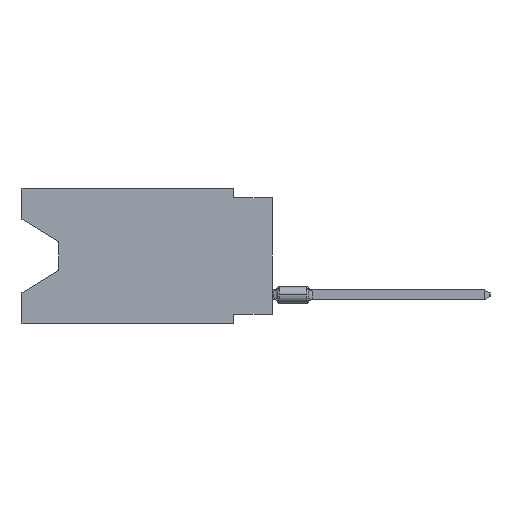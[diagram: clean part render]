
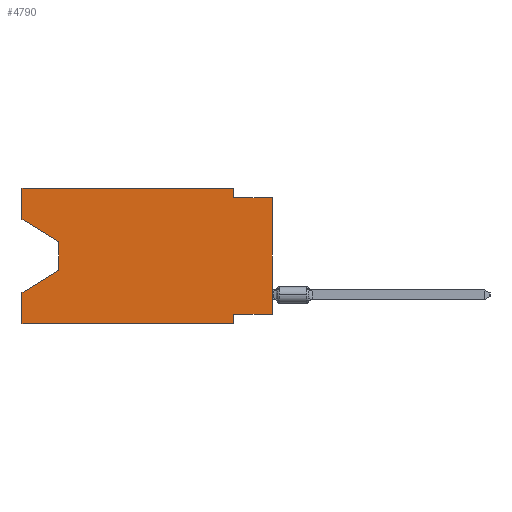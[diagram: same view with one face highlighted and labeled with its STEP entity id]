
A CAD part, left-side view. The second image highlights one B-rep face of the part: STEP entity #4790.
In plain terms, the highlighted planar face has unit normal (-1, 0, 0).
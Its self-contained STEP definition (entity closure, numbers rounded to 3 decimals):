
#1684 = DIRECTION ( 'NONE',  ( 0., -1., 0. ) ) ;
#2310 = VECTOR ( 'NONE', #32259, 1000. ) ;
#2344 = VERTEX_POINT ( 'NONE', #59910 ) ;
#2528 = CARTESIAN_POINT ( 'NONE',  ( 0., 16.383, 0. ) ) ;
#3266 = CARTESIAN_POINT ( 'NONE',  ( 0., 16.383, 0. ) ) ;
#3654 = CARTESIAN_POINT ( 'NONE',  ( 0., 16.383, 0. ) ) ;
#3919 = DIRECTION ( 'NONE',  ( 0., 0., 1. ) ) ;
#4790 = ADVANCED_FACE ( 'NONE', ( #25564 ), #44043, .F. ) ;
#5219 = ORIENTED_EDGE ( 'NONE', *, *, #53636, .F. ) ;
#5484 = VECTOR ( 'NONE', #18317, 1000. ) ;
#5953 = VERTEX_POINT ( 'NONE', #3266 ) ;
#6232 = LINE ( 'NONE', #38947, #46219 ) ;
#6606 = VERTEX_POINT ( 'NONE', #14410 ) ;
#6615 = CARTESIAN_POINT ( 'NONE',  ( 0., 16.383, 0. ) ) ;
#6878 = ORIENTED_EDGE ( 'NONE', *, *, #52395, .F. ) ;
#7997 = DIRECTION ( 'NONE',  ( 0., 1., 0. ) ) ;
#8465 = VERTEX_POINT ( 'NONE', #28831 ) ;
#8543 = CARTESIAN_POINT ( 'NONE',  ( 0., 2.54, -0.635 ) ) ;
#8695 = VECTOR ( 'NONE', #53645, 1000. ) ;
#8993 = CARTESIAN_POINT ( 'NONE',  ( 0., 16.383, 0. ) ) ;
#9482 = DIRECTION ( 'NONE',  ( 0., -0.855, -0.519 ) ) ;
#9536 = VECTOR ( 'NONE', #13551, 1000. ) ;
#10399 = ORIENTED_EDGE ( 'NONE', *, *, #22280, .T. ) ;
#10904 = ORIENTED_EDGE ( 'NONE', *, *, #12174, .F. ) ;
#11499 = VECTOR ( 'NONE', #42005, 1000. ) ;
#11613 = AXIS2_PLACEMENT_3D ( 'NONE', #2528, #21022, #39489 ) ;
#12174 = EDGE_CURVE ( 'NONE', #33151, #37188, #49015, .T. ) ;
#12844 = LINE ( 'NONE', #54327, #21352 ) ;
#13045 = LINE ( 'NONE', #3654, #8695 ) ;
#13262 = CARTESIAN_POINT ( 'NONE',  ( 0., 16.383, -2.038 ) ) ;
#13551 = DIRECTION ( 'NONE',  ( 0., 0.855, -0.519 ) ) ;
#14410 = CARTESIAN_POINT ( 'NONE',  ( 0., 0., -8.255 ) ) ;
#15656 = CARTESIAN_POINT ( 'NONE',  ( 0., 0., -0.635 ) ) ;
#16325 = DIRECTION ( 'NONE',  ( 0., 0., 1. ) ) ;
#16376 = ORIENTED_EDGE ( 'NONE', *, *, #46644, .F. ) ;
#18317 = DIRECTION ( 'NONE',  ( 0., 0., -1. ) ) ;
#18610 = CARTESIAN_POINT ( 'NONE',  ( 0., 2.54, 0. ) ) ;
#19318 = ORIENTED_EDGE ( 'NONE', *, *, #20815, .F. ) ;
#20003 = VERTEX_POINT ( 'NONE', #24184 ) ;
#20815 = EDGE_CURVE ( 'NONE', #23128, #49265, #54342, .T. ) ;
#21022 = DIRECTION ( 'NONE',  ( 1., 0., 0. ) ) ;
#21352 = VECTOR ( 'NONE', #7997, 1000. ) ;
#22280 = EDGE_CURVE ( 'NONE', #33151, #55894, #6232, .T. ) ;
#22934 = CARTESIAN_POINT ( 'NONE',  ( 0., 13.97, -5.385 ) ) ;
#23128 = VERTEX_POINT ( 'NONE', #39033 ) ;
#23305 = EDGE_CURVE ( 'NONE', #20003, #37188, #35682, .T. ) ;
#23822 = EDGE_LOOP ( 'NONE', ( #55462, #25650, #25593, #10904, #10399, #5219, #50854, #59811, #6878, #19318, #16376, #44532 ) ) ;
#24184 = CARTESIAN_POINT ( 'NONE',  ( 0., 13.97, -5.385 ) ) ;
#25208 = VERTEX_POINT ( 'NONE', #42672 ) ;
#25564 = FACE_OUTER_BOUND ( 'NONE', #23822, .T. ) ;
#25593 = ORIENTED_EDGE ( 'NONE', *, *, #23305, .T. ) ;
#25650 = ORIENTED_EDGE ( 'NONE', *, *, #45977, .T. ) ;
#26534 = LINE ( 'NONE', #50130, #2310 ) ;
#28284 = CARTESIAN_POINT ( 'NONE',  ( 0., 13.97, -3.505 ) ) ;
#28831 = CARTESIAN_POINT ( 'NONE',  ( 0., 0., -0.635 ) ) ;
#30468 = DIRECTION ( 'NONE',  ( 0., -1., 0. ) ) ;
#32259 = DIRECTION ( 'NONE',  ( 0., 0., -1. ) ) ;
#32826 = LINE ( 'NONE', #28284, #38567 ) ;
#33095 = CARTESIAN_POINT ( 'NONE',  ( 0., 16.383, -2.038 ) ) ;
#33151 = VERTEX_POINT ( 'NONE', #34216 ) ;
#34216 = CARTESIAN_POINT ( 'NONE',  ( 0., 16.383, -8.89 ) ) ;
#35682 = LINE ( 'NONE', #22934, #9536 ) ;
#36032 = CARTESIAN_POINT ( 'NONE',  ( 0., 0., 0. ) ) ;
#36073 = EDGE_CURVE ( 'NONE', #54749, #5953, #13045, .T. ) ;
#37188 = VERTEX_POINT ( 'NONE', #53187 ) ;
#38567 = VECTOR ( 'NONE', #51593, 1000. ) ;
#38947 = CARTESIAN_POINT ( 'NONE',  ( 0., 16.383, -8.89 ) ) ;
#39033 = CARTESIAN_POINT ( 'NONE',  ( 0., 2.54, 0. ) ) ;
#39489 = DIRECTION ( 'NONE',  ( 0., 0., -1. ) ) ;
#42005 = DIRECTION ( 'NONE',  ( 0., -1., 0. ) ) ;
#42093 = VECTOR ( 'NONE', #16325, 1000. ) ;
#42513 = VECTOR ( 'NONE', #9482, 1000. ) ;
#42672 = CARTESIAN_POINT ( 'NONE',  ( 0., 2.54, -8.255 ) ) ;
#43217 = LINE ( 'NONE', #15656, #49612 ) ;
#43381 = CARTESIAN_POINT ( 'NONE',  ( 0., 2.54, -8.89 ) ) ;
#44043 = PLANE ( 'NONE',  #11613 ) ;
#44532 = ORIENTED_EDGE ( 'NONE', *, *, #36073, .F. ) ;
#44556 = LINE ( 'NONE', #36032, #51992 ) ;
#44920 = EDGE_CURVE ( 'NONE', #6606, #8465, #44556, .T. ) ;
#45977 = EDGE_CURVE ( 'NONE', #2344, #20003, #32826, .T. ) ;
#46219 = VECTOR ( 'NONE', #1684, 1000. ) ;
#46546 = LINE ( 'NONE', #8993, #11499 ) ;
#46644 = EDGE_CURVE ( 'NONE', #5953, #23128, #46546, .T. ) ;
#46888 = EDGE_CURVE ( 'NONE', #54749, #2344, #50377, .T. ) ;
#49015 = LINE ( 'NONE', #6615, #42093 ) ;
#49265 = VERTEX_POINT ( 'NONE', #8543 ) ;
#49612 = VECTOR ( 'NONE', #30468, 1000. ) ;
#50130 = CARTESIAN_POINT ( 'NONE',  ( 0., 2.54, -8.89 ) ) ;
#50377 = LINE ( 'NONE', #33095, #42513 ) ;
#50854 = ORIENTED_EDGE ( 'NONE', *, *, #58614, .F. ) ;
#51593 = DIRECTION ( 'NONE',  ( 0., 0., -1. ) ) ;
#51992 = VECTOR ( 'NONE', #3919, 1000. ) ;
#52395 = EDGE_CURVE ( 'NONE', #49265, #8465, #43217, .T. ) ;
#53187 = CARTESIAN_POINT ( 'NONE',  ( 0., 16.383, -6.852 ) ) ;
#53636 = EDGE_CURVE ( 'NONE', #25208, #55894, #26534, .T. ) ;
#53645 = DIRECTION ( 'NONE',  ( 0., 0., 1. ) ) ;
#54327 = CARTESIAN_POINT ( 'NONE',  ( 0., 0., -8.255 ) ) ;
#54342 = LINE ( 'NONE', #18610, #5484 ) ;
#54749 = VERTEX_POINT ( 'NONE', #13262 ) ;
#55462 = ORIENTED_EDGE ( 'NONE', *, *, #46888, .T. ) ;
#55894 = VERTEX_POINT ( 'NONE', #43381 ) ;
#58614 = EDGE_CURVE ( 'NONE', #6606, #25208, #12844, .T. ) ;
#59811 = ORIENTED_EDGE ( 'NONE', *, *, #44920, .T. ) ;
#59910 = CARTESIAN_POINT ( 'NONE',  ( 0., 13.97, -3.505 ) ) ;
